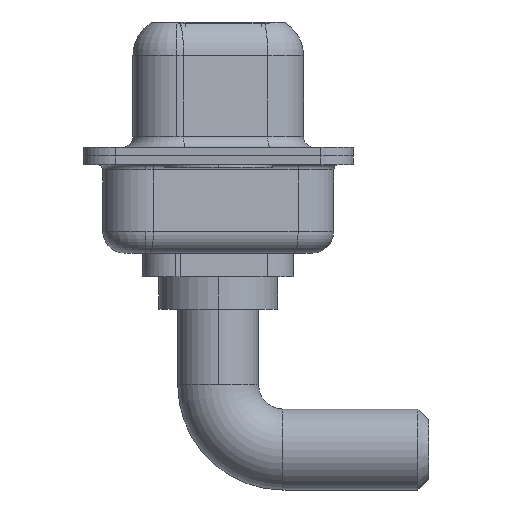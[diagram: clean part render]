
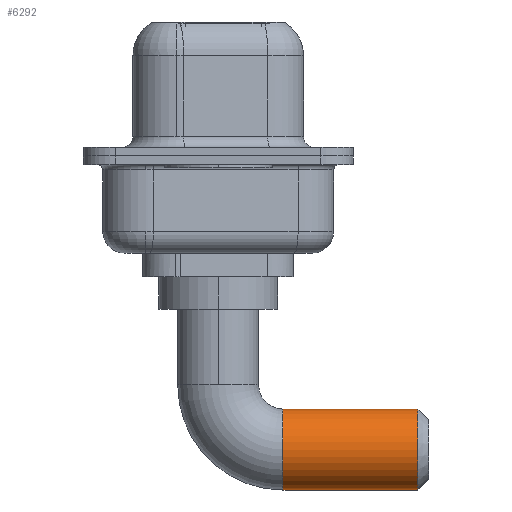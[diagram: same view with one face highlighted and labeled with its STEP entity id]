
A CAD part, left-side view. The second image highlights one B-rep face of the part: STEP entity #6292.
In plain terms, the highlighted cylindrical face has radius 1.875 mm (diameter 3.75 mm), a partial arc.
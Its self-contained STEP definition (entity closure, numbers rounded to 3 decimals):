
#64 = EDGE_CURVE ( 'NONE', #7488, #5461, #3541, .T. ) ;
#229 = FACE_OUTER_BOUND ( 'NONE', #4679, .T. ) ;
#247 = DIRECTION ( 'NONE',  ( 0., -1., 0. ) ) ;
#287 = CARTESIAN_POINT ( 'NONE',  ( 0., -3., -6.5 ) ) ;
#318 = EDGE_CURVE ( 'NONE', #1673, #9079, #8831, .T. ) ;
#407 = VECTOR ( 'NONE', #10923, 1000. ) ;
#610 = DIRECTION ( 'NONE',  ( 0., -1., 0. ) ) ;
#684 = CARTESIAN_POINT ( 'NONE',  ( 0., -9.25, -4.625 ) ) ;
#840 = CARTESIAN_POINT ( 'NONE',  ( 0., -3., -4.625 ) ) ;
#1673 = VERTEX_POINT ( 'NONE', #9824 ) ;
#2349 = DIRECTION ( 'NONE',  ( 0., 0., -1. ) ) ;
#2803 = DIRECTION ( 'NONE',  ( -1., 0., 0. ) ) ;
#2840 = DIRECTION ( 'NONE',  ( 0., 0., -1. ) ) ;
#2858 = CARTESIAN_POINT ( 'NONE',  ( 0., -3., -6.5 ) ) ;
#3036 = CARTESIAN_POINT ( 'NONE',  ( 0., -9.25, -6.5 ) ) ;
#3189 = AXIS2_PLACEMENT_3D ( 'NONE', #2858, #247, #2803 ) ;
#3541 = CIRCLE ( 'NONE', #10061, 1.875 ) ;
#3672 = DIRECTION ( 'NONE',  ( 0., -1., 0. ) ) ;
#4196 = LINE ( 'NONE', #7574, #407 ) ;
#4679 = EDGE_LOOP ( 'NONE', ( #10245, #6735, #8523, #5892 ) ) ;
#4974 = DIRECTION ( 'NONE',  ( 0., 1., 0. ) ) ;
#5461 = VERTEX_POINT ( 'NONE', #684 ) ;
#5892 = ORIENTED_EDGE ( 'NONE', *, *, #64, .T. ) ;
#6292 = ADVANCED_FACE ( 'NONE', ( #229 ), #7874, .T. ) ;
#6735 = ORIENTED_EDGE ( 'NONE', *, *, #318, .T. ) ;
#6890 = EDGE_CURVE ( 'NONE', #9079, #7488, #4196, .T. ) ;
#7018 = VECTOR ( 'NONE', #610, 1000. ) ;
#7116 = CARTESIAN_POINT ( 'NONE',  ( 0., -3., -8.375 ) ) ;
#7488 = VERTEX_POINT ( 'NONE', #10298 ) ;
#7574 = CARTESIAN_POINT ( 'NONE',  ( 0., -3., -8.375 ) ) ;
#7874 = CYLINDRICAL_SURFACE ( 'NONE', #9264, 1.875 ) ;
#8523 = ORIENTED_EDGE ( 'NONE', *, *, #6890, .T. ) ;
#8831 = CIRCLE ( 'NONE', #3189, 1.875 ) ;
#9079 = VERTEX_POINT ( 'NONE', #7116 ) ;
#9264 = AXIS2_PLACEMENT_3D ( 'NONE', #287, #3672, #2840 ) ;
#9533 = EDGE_CURVE ( 'NONE', #1673, #5461, #10846, .T. ) ;
#9824 = CARTESIAN_POINT ( 'NONE',  ( 0., -3., -4.625 ) ) ;
#10061 = AXIS2_PLACEMENT_3D ( 'NONE', #3036, #4974, #2349 ) ;
#10245 = ORIENTED_EDGE ( 'NONE', *, *, #9533, .F. ) ;
#10298 = CARTESIAN_POINT ( 'NONE',  ( 0., -9.25, -8.375 ) ) ;
#10846 = LINE ( 'NONE', #840, #7018 ) ;
#10923 = DIRECTION ( 'NONE',  ( 0., -1., 0. ) ) ;
